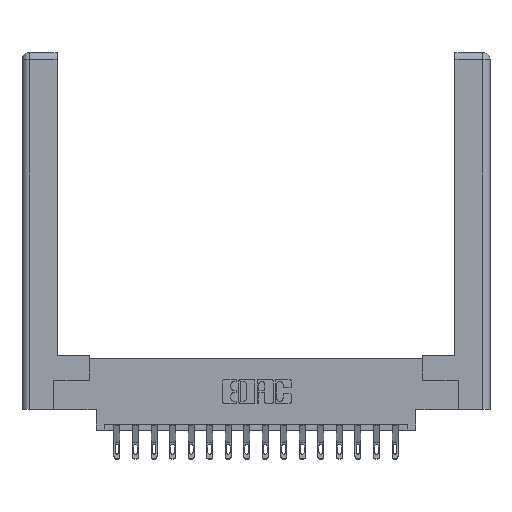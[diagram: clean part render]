
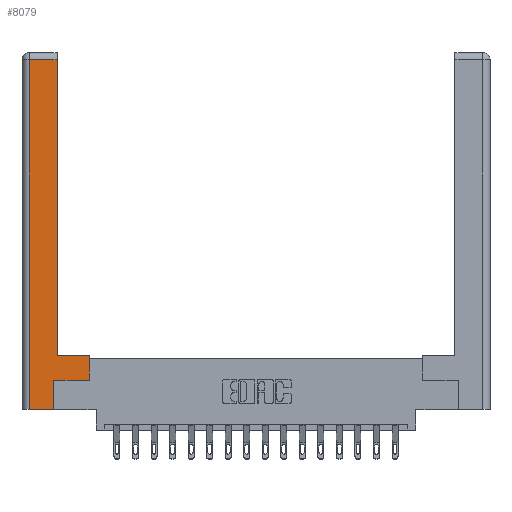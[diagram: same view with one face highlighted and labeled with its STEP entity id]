
A CAD part, top view. The second image highlights one B-rep face of the part: STEP entity #8079.
In plain terms, the highlighted planar face has unit normal (0, 0, 1).
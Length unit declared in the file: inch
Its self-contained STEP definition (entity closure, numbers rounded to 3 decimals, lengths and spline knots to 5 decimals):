
#29 = LINE ( 'NONE', #11699, #17590 ) ;
#149 = CARTESIAN_POINT ( 'NONE',  ( 0.265, 0., 0. ) ) ;
#441 = ORIENTED_EDGE ( 'NONE', *, *, #9770, .T. ) ;
#702 = DIRECTION ( 'NONE',  ( -1., 0., 0. ) ) ;
#1215 = VECTOR ( 'NONE', #15904, 39.37008 ) ;
#1380 = VERTEX_POINT ( 'NONE', #6841 ) ;
#1610 = VECTOR ( 'NONE', #1637, 39.37008 ) ;
#1637 = DIRECTION ( 'NONE',  ( -1., 0., 0. ) ) ;
#1785 = VERTEX_POINT ( 'NONE', #8315 ) ;
#1793 = VECTOR ( 'NONE', #6677, 39.37008 ) ;
#2372 = LINE ( 'NONE', #3150, #17403 ) ;
#2408 = CARTESIAN_POINT ( 'NONE',  ( 0.295, 0.45, 0. ) ) ;
#3092 = EDGE_CURVE ( 'NONE', #17515, #15713, #11765, .T. ) ;
#3150 = CARTESIAN_POINT ( 'NONE',  ( 0.265, 0., 0. ) ) ;
#3265 = DIRECTION ( 'NONE',  ( 1., 0., 0. ) ) ;
#3292 = ORIENTED_EDGE ( 'NONE', *, *, #12082, .T. ) ;
#3501 = CARTESIAN_POINT ( 'NONE',  ( 0., 0., 0. ) ) ;
#3715 = LINE ( 'NONE', #2408, #3935 ) ;
#3935 = VECTOR ( 'NONE', #702, 39.37008 ) ;
#4056 = EDGE_LOOP ( 'NONE', ( #18415, #18074, #13552, #9590, #18171, #3292, #18070, #441 ) ) ;
#4105 = LINE ( 'NONE', #10465, #1610 ) ;
#4800 = VERTEX_POINT ( 'NONE', #9344 ) ;
#5079 = CARTESIAN_POINT ( 'NONE',  ( 0.565, 0.245, 0. ) ) ;
#5363 = VERTEX_POINT ( 'NONE', #149 ) ;
#5905 = CARTESIAN_POINT ( 'NONE',  ( 0.0615, 0., 0. ) ) ;
#6106 = DIRECTION ( 'NONE',  ( 0., 1., 0. ) ) ;
#6491 = FACE_OUTER_BOUND ( 'NONE', #4056, .T. ) ;
#6677 = DIRECTION ( 'NONE',  ( 1., 0., 0. ) ) ;
#6841 = CARTESIAN_POINT ( 'NONE',  ( 0.0615, 2.94, 0. ) ) ;
#6990 = DIRECTION ( 'NONE',  ( 0., 1., 0. ) ) ;
#7214 = CARTESIAN_POINT ( 'NONE',  ( 0.0615, 0., 0. ) ) ;
#7607 = EDGE_CURVE ( 'NONE', #15973, #5363, #2372, .T. ) ;
#7628 = CARTESIAN_POINT ( 'NONE',  ( 0.265, 0.245, 0. ) ) ;
#8079 = ADVANCED_FACE ( 'NONE', ( #6491 ), #12445, .F. ) ;
#8315 = CARTESIAN_POINT ( 'NONE',  ( 0.295, 0.45, 0. ) ) ;
#8442 = EDGE_CURVE ( 'NONE', #1380, #15973, #13101, .T. ) ;
#9344 = CARTESIAN_POINT ( 'NONE',  ( 0.295, 2.94, 0. ) ) ;
#9541 = CARTESIAN_POINT ( 'NONE',  ( 0.565, 0.45, 0. ) ) ;
#9587 = LINE ( 'NONE', #5079, #1793 ) ;
#9590 = ORIENTED_EDGE ( 'NONE', *, *, #7607, .T. ) ;
#9634 = CARTESIAN_POINT ( 'NONE',  ( 0.565, 0.245, 0. ) ) ;
#9770 = EDGE_CURVE ( 'NONE', #15713, #1785, #3715, .T. ) ;
#10071 = LINE ( 'NONE', #7628, #17602 ) ;
#10329 = EDGE_CURVE ( 'NONE', #1785, #4800, #29, .T. ) ;
#10465 = CARTESIAN_POINT ( 'NONE',  ( 0.0615, 2.94, 0. ) ) ;
#11699 = CARTESIAN_POINT ( 'NONE',  ( 0.295, 3., 0. ) ) ;
#11765 = LINE ( 'NONE', #18803, #12249 ) ;
#12082 = EDGE_CURVE ( 'NONE', #18316, #17515, #9587, .T. ) ;
#12249 = VECTOR ( 'NONE', #6990, 39.37008 ) ;
#12445 = PLANE ( 'NONE',  #13481 ) ;
#13101 = LINE ( 'NONE', #7214, #1215 ) ;
#13481 = AXIS2_PLACEMENT_3D ( 'NONE', #3501, #15279, #18112 ) ;
#13552 = ORIENTED_EDGE ( 'NONE', *, *, #8442, .T. ) ;
#14289 = CARTESIAN_POINT ( 'NONE',  ( 0.265, 0.245, 0. ) ) ;
#14679 = DIRECTION ( 'NONE',  ( 0., 1., 0. ) ) ;
#14721 = EDGE_CURVE ( 'NONE', #5363, #18316, #10071, .T. ) ;
#15279 = DIRECTION ( 'NONE',  ( 0., 0., -1. ) ) ;
#15713 = VERTEX_POINT ( 'NONE', #9541 ) ;
#15904 = DIRECTION ( 'NONE',  ( 0., -1., 0. ) ) ;
#15973 = VERTEX_POINT ( 'NONE', #5905 ) ;
#15977 = EDGE_CURVE ( 'NONE', #4800, #1380, #4105, .T. ) ;
#17403 = VECTOR ( 'NONE', #3265, 39.37008 ) ;
#17515 = VERTEX_POINT ( 'NONE', #9634 ) ;
#17590 = VECTOR ( 'NONE', #14679, 39.37008 ) ;
#17602 = VECTOR ( 'NONE', #6106, 39.37008 ) ;
#18070 = ORIENTED_EDGE ( 'NONE', *, *, #3092, .T. ) ;
#18074 = ORIENTED_EDGE ( 'NONE', *, *, #15977, .T. ) ;
#18112 = DIRECTION ( 'NONE',  ( -1., 0., 0. ) ) ;
#18171 = ORIENTED_EDGE ( 'NONE', *, *, #14721, .T. ) ;
#18316 = VERTEX_POINT ( 'NONE', #14289 ) ;
#18415 = ORIENTED_EDGE ( 'NONE', *, *, #10329, .T. ) ;
#18803 = CARTESIAN_POINT ( 'NONE',  ( 0.565, 0.45, 0. ) ) ;
